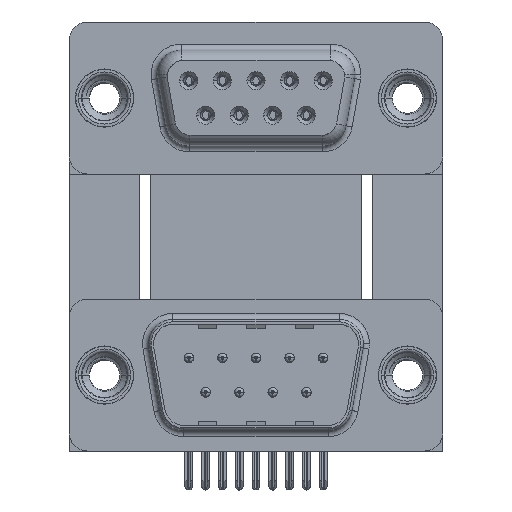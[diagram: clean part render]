
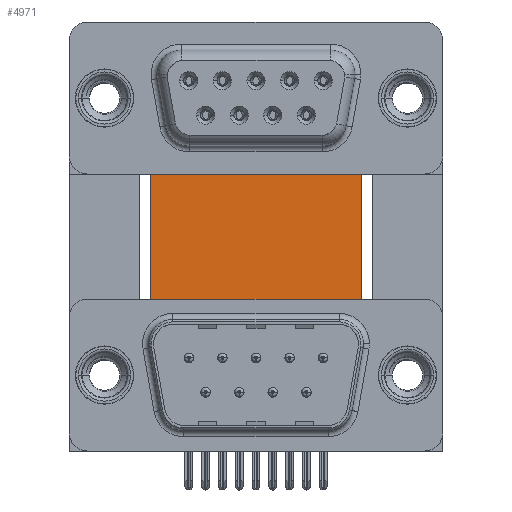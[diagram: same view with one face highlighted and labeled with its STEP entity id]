
A CAD part, top view. The second image highlights one B-rep face of the part: STEP entity #4971.
In plain terms, the highlighted planar face has unit normal (0, 0, 1).
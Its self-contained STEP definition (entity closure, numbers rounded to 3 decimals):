
#233 = LINE ( 'NONE', #12479, #22203 ) ;
#632 = LINE ( 'NONE', #30391, #10193 ) ;
#651 = LINE ( 'NONE', #3464, #1817 ) ;
#892 = VECTOR ( 'NONE', #16371, 1000. ) ;
#1817 = VECTOR ( 'NONE', #3659, 1000. ) ;
#2924 = VECTOR ( 'NONE', #26916, 1000. ) ;
#2942 = ORIENTED_EDGE ( 'NONE', *, *, #24078, .F. ) ;
#3433 = VERTEX_POINT ( 'NONE', #4177 ) ;
#3464 = CARTESIAN_POINT ( 'NONE',  ( 22.59, -4.635, -12. ) ) ;
#3659 = DIRECTION ( 'NONE',  ( -0.336, 0.942, 0. ) ) ;
#3712 = VECTOR ( 'NONE', #9089, 1000. ) ;
#4177 = CARTESIAN_POINT ( 'NONE',  ( 22.59, -4.635, -12. ) ) ;
#4219 = LINE ( 'NONE', #5409, #2924 ) ;
#4971 = ADVANCED_FACE ( 'NONE', ( #32492 ), #10749, .F. ) ;
#5230 = DIRECTION ( 'NONE',  ( 1., 0., 0. ) ) ;
#5409 = CARTESIAN_POINT ( 'NONE',  ( 3.79, 16.585, -12. ) ) ;
#6188 = VERTEX_POINT ( 'NONE', #36479 ) ;
#7097 = LINE ( 'NONE', #37503, #892 ) ;
#7723 = CARTESIAN_POINT ( 'NONE',  ( 21.2, -0.735, -12. ) ) ;
#7734 = CARTESIAN_POINT ( 'NONE',  ( 3.79, 16.585, -12. ) ) ;
#8131 = DIRECTION ( 'NONE',  ( 0., 0., -1. ) ) ;
#8197 = VERTEX_POINT ( 'NONE', #23099 ) ;
#9089 = DIRECTION ( 'NONE',  ( 0., -1., 0. ) ) ;
#10193 = VECTOR ( 'NONE', #27375, 1000. ) ;
#10343 = CARTESIAN_POINT ( 'NONE',  ( 3.79, 16.585, -12. ) ) ;
#10601 = VECTOR ( 'NONE', #31874, 1000. ) ;
#10749 = PLANE ( 'NONE',  #38487 ) ;
#12129 = ORIENTED_EDGE ( 'NONE', *, *, #22480, .T. ) ;
#12301 = CARTESIAN_POINT ( 'NONE',  ( 22.09, -3.735, -12. ) ) ;
#12304 = EDGE_CURVE ( 'NONE', #6188, #14787, #4219, .T. ) ;
#12479 = CARTESIAN_POINT ( 'NONE',  ( 2.9, -4.635, -12. ) ) ;
#13551 = LINE ( 'NONE', #38099, #28581 ) ;
#13555 = ORIENTED_EDGE ( 'NONE', *, *, #12304, .F. ) ;
#14787 = VERTEX_POINT ( 'NONE', #35771 ) ;
#15943 = ORIENTED_EDGE ( 'NONE', *, *, #37250, .T. ) ;
#15965 = LINE ( 'NONE', #28808, #22067 ) ;
#16371 = DIRECTION ( 'NONE',  ( 0., 1., 0. ) ) ;
#16444 = CARTESIAN_POINT ( 'NONE',  ( 2.9, -3.735, -12. ) ) ;
#17522 = EDGE_CURVE ( 'NONE', #6188, #8197, #34507, .T. ) ;
#17531 = EDGE_CURVE ( 'NONE', #28444, #22077, #13551, .T. ) ;
#17607 = ORIENTED_EDGE ( 'NONE', *, *, #17531, .T. ) ;
#17660 = VERTEX_POINT ( 'NONE', #7723 ) ;
#17701 = CARTESIAN_POINT ( 'NONE',  ( 22.09, -4.635, -12. ) ) ;
#17972 = ORIENTED_EDGE ( 'NONE', *, *, #17522, .T. ) ;
#18716 = DIRECTION ( 'NONE',  ( 1., 0., 0. ) ) ;
#22067 = VECTOR ( 'NONE', #37871, 1000. ) ;
#22077 = VERTEX_POINT ( 'NONE', #27940 ) ;
#22156 = LINE ( 'NONE', #12301, #3712 ) ;
#22203 = VECTOR ( 'NONE', #18716, 1000. ) ;
#22480 = EDGE_CURVE ( 'NONE', #33976, #28444, #7097, .T. ) ;
#22815 = DIRECTION ( 'NONE',  ( 1., 0., 0. ) ) ;
#23099 = CARTESIAN_POINT ( 'NONE',  ( 3.79, -0.735, -12. ) ) ;
#23923 = LINE ( 'NONE', #17701, #36488 ) ;
#24078 = EDGE_CURVE ( 'NONE', #14787, #17660, #15965, .T. ) ;
#24447 = ORIENTED_EDGE ( 'NONE', *, *, #32886, .T. ) ;
#25817 = ORIENTED_EDGE ( 'NONE', *, *, #27028, .T. ) ;
#26916 = DIRECTION ( 'NONE',  ( 1., 0., 0. ) ) ;
#27028 = EDGE_CURVE ( 'NONE', #27590, #33976, #233, .T. ) ;
#27375 = DIRECTION ( 'NONE',  ( -0.336, -0.942, 0. ) ) ;
#27590 = VERTEX_POINT ( 'NONE', #30292 ) ;
#27940 = CARTESIAN_POINT ( 'NONE',  ( 22.09, -3.735, -12. ) ) ;
#28444 = VERTEX_POINT ( 'NONE', #16444 ) ;
#28581 = VECTOR ( 'NONE', #22815, 1000. ) ;
#28620 = CARTESIAN_POINT ( 'NONE',  ( 22.09, -4.635, -12. ) ) ;
#28808 = CARTESIAN_POINT ( 'NONE',  ( 21.2, 16.585, -12. ) ) ;
#30292 = CARTESIAN_POINT ( 'NONE',  ( 2.4, -4.635, -12. ) ) ;
#30377 = ORIENTED_EDGE ( 'NONE', *, *, #37418, .T. ) ;
#30391 = CARTESIAN_POINT ( 'NONE',  ( 2.4, -4.635, -12. ) ) ;
#31874 = DIRECTION ( 'NONE',  ( 0., -1., 0. ) ) ;
#31887 = DIRECTION ( 'NONE',  ( -1., 0., 0. ) ) ;
#32492 = FACE_OUTER_BOUND ( 'NONE', #39197, .T. ) ;
#32886 = EDGE_CURVE ( 'NONE', #8197, #27590, #632, .T. ) ;
#33976 = VERTEX_POINT ( 'NONE', #34849 ) ;
#34005 = ORIENTED_EDGE ( 'NONE', *, *, #39521, .T. ) ;
#34507 = LINE ( 'NONE', #10343, #10601 ) ;
#34849 = CARTESIAN_POINT ( 'NONE',  ( 2.9, -4.635, -12. ) ) ;
#35771 = CARTESIAN_POINT ( 'NONE',  ( 21.2, 16.585, -12. ) ) ;
#36479 = CARTESIAN_POINT ( 'NONE',  ( 3.79, 16.585, -12. ) ) ;
#36488 = VECTOR ( 'NONE', #5230, 1000. ) ;
#37250 = EDGE_CURVE ( 'NONE', #22077, #39250, #22156, .T. ) ;
#37418 = EDGE_CURVE ( 'NONE', #39250, #3433, #23923, .T. ) ;
#37503 = CARTESIAN_POINT ( 'NONE',  ( 2.9, -3.735, -12. ) ) ;
#37871 = DIRECTION ( 'NONE',  ( 0., -1., 0. ) ) ;
#38099 = CARTESIAN_POINT ( 'NONE',  ( 3.79, -3.735, -12. ) ) ;
#38487 = AXIS2_PLACEMENT_3D ( 'NONE', #7734, #8131, #31887 ) ;
#39197 = EDGE_LOOP ( 'NONE', ( #17607, #15943, #30377, #34005, #2942, #13555, #17972, #24447, #25817, #12129 ) ) ;
#39250 = VERTEX_POINT ( 'NONE', #28620 ) ;
#39521 = EDGE_CURVE ( 'NONE', #3433, #17660, #651, .T. ) ;
